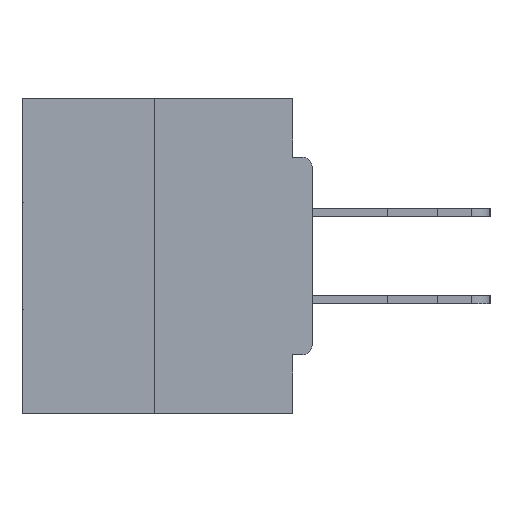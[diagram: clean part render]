
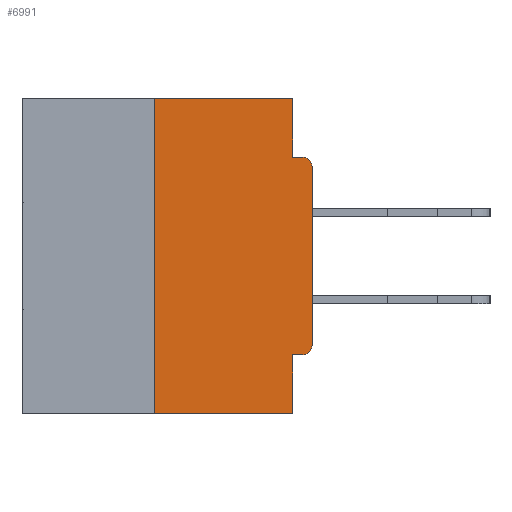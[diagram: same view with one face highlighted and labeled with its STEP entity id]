
A CAD part, left-side view. The second image highlights one B-rep face of the part: STEP entity #6991.
In plain terms, the highlighted planar face has unit normal (-1, 0, 0).
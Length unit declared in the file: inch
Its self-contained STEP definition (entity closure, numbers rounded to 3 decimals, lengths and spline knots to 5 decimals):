
#380 = CIRCLE ( 'NONE', #31904, 0.015 ) ;
#1742 = DIRECTION ( 'NONE',  ( 0., -1., 0. ) ) ;
#1920 = CARTESIAN_POINT ( 'NONE',  ( 0., 0.25, 0. ) ) ;
#2111 = DIRECTION ( 'NONE',  ( 0., 0., -1. ) ) ;
#2274 = LINE ( 'NONE', #31987, #38668 ) ;
#2423 = EDGE_CURVE ( 'NONE', #7994, #30855, #2274, .T. ) ;
#3061 = CARTESIAN_POINT ( 'NONE',  ( 0., 0., -0.4065 ) ) ;
#3167 = ORIENTED_EDGE ( 'NONE', *, *, #2423, .F. ) ;
#3292 = VERTEX_POINT ( 'NONE', #24908 ) ;
#3444 = ORIENTED_EDGE ( 'NONE', *, *, #24494, .T. ) ;
#4400 = EDGE_CURVE ( 'NONE', #24408, #22154, #13901, .T. ) ;
#4597 = CARTESIAN_POINT ( 'NONE',  ( 0., 0.46, -0.5 ) ) ;
#5049 = LINE ( 'NONE', #6935, #36256 ) ;
#5196 = CARTESIAN_POINT ( 'NONE',  ( 0., 0.015, -0.1085 ) ) ;
#6489 = AXIS2_PLACEMENT_3D ( 'NONE', #35710, #23314, #20119 ) ;
#6546 = CARTESIAN_POINT ( 'NONE',  ( 0., 0.031, 0. ) ) ;
#6935 = CARTESIAN_POINT ( 'NONE',  ( 0., 0.031, -0.5 ) ) ;
#6991 = ADVANCED_FACE ( 'NONE', ( #25486 ), #13376, .F. ) ;
#7063 = LINE ( 'NONE', #1920, #12255 ) ;
#7415 = EDGE_CURVE ( 'NONE', #3292, #23061, #25901, .T. ) ;
#7994 = VERTEX_POINT ( 'NONE', #30016 ) ;
#8171 = CARTESIAN_POINT ( 'NONE',  ( 0., 0.031, 0. ) ) ;
#8241 = CARTESIAN_POINT ( 'NONE',  ( 0., 0., -0.1085 ) ) ;
#8662 = VERTEX_POINT ( 'NONE', #27931 ) ;
#9055 = EDGE_LOOP ( 'NONE', ( #31337, #34740, #13455, #33193, #10926, #36842, #31069, #3444, #3167, #16853 ) ) ;
#9087 = EDGE_CURVE ( 'NONE', #8662, #24222, #30513, .T. ) ;
#9324 = EDGE_CURVE ( 'NONE', #22154, #23061, #5049, .T. ) ;
#10466 = DIRECTION ( 'NONE',  ( 0., 0., -1. ) ) ;
#10768 = CIRCLE ( 'NONE', #6489, 0.015 ) ;
#10926 = ORIENTED_EDGE ( 'NONE', *, *, #4400, .F. ) ;
#11288 = DIRECTION ( 'NONE',  ( -1., 0., 0. ) ) ;
#12234 = CARTESIAN_POINT ( 'NONE',  ( 0., 0.46, 0. ) ) ;
#12255 = VECTOR ( 'NONE', #34930, 39.37008 ) ;
#13376 = PLANE ( 'NONE',  #23803 ) ;
#13455 = ORIENTED_EDGE ( 'NONE', *, *, #7415, .T. ) ;
#13722 = VERTEX_POINT ( 'NONE', #32811 ) ;
#13901 = LINE ( 'NONE', #3061, #38012 ) ;
#14925 = DIRECTION ( 'NONE',  ( 0., 0., 1. ) ) ;
#15046 = CARTESIAN_POINT ( 'NONE',  ( 0., 0., 0. ) ) ;
#16214 = VECTOR ( 'NONE', #14925, 39.37008 ) ;
#16529 = CARTESIAN_POINT ( 'NONE',  ( 0., 0.46, 0. ) ) ;
#16853 = ORIENTED_EDGE ( 'NONE', *, *, #37909, .F. ) ;
#17855 = CARTESIAN_POINT ( 'NONE',  ( 0., 0.015, -0.0935 ) ) ;
#20119 = DIRECTION ( 'NONE',  ( 0., 0., -1. ) ) ;
#20407 = DIRECTION ( 'NONE',  ( 0., 0., -1. ) ) ;
#21419 = EDGE_CURVE ( 'NONE', #24408, #13722, #10768, .T. ) ;
#21556 = VECTOR ( 'NONE', #35613, 39.37008 ) ;
#22020 = CARTESIAN_POINT ( 'NONE',  ( 0., 0.015, -0.4065 ) ) ;
#22154 = VERTEX_POINT ( 'NONE', #23844 ) ;
#23061 = VERTEX_POINT ( 'NONE', #35053 ) ;
#23314 = DIRECTION ( 'NONE',  ( -1., 0., 0. ) ) ;
#23803 = AXIS2_PLACEMENT_3D ( 'NONE', #16529, #25124, #10466 ) ;
#23844 = CARTESIAN_POINT ( 'NONE',  ( 0., 0.031, -0.4065 ) ) ;
#24222 = VERTEX_POINT ( 'NONE', #6546 ) ;
#24339 = EDGE_CURVE ( 'NONE', #3292, #8662, #7063, .T. ) ;
#24408 = VERTEX_POINT ( 'NONE', #22020 ) ;
#24494 = EDGE_CURVE ( 'NONE', #27863, #30855, #380, .T. ) ;
#24908 = CARTESIAN_POINT ( 'NONE',  ( 0., 0.25, -0.5 ) ) ;
#25124 = DIRECTION ( 'NONE',  ( 1., 0., 0. ) ) ;
#25139 = DIRECTION ( 'NONE',  ( 0., 0., -1. ) ) ;
#25388 = LINE ( 'NONE', #8171, #37705 ) ;
#25486 = FACE_OUTER_BOUND ( 'NONE', #9055, .T. ) ;
#25841 = DIRECTION ( 'NONE',  ( 0., -1., 0. ) ) ;
#25901 = LINE ( 'NONE', #4597, #26394 ) ;
#26394 = VECTOR ( 'NONE', #25841, 39.37008 ) ;
#27863 = VERTEX_POINT ( 'NONE', #8241 ) ;
#27931 = CARTESIAN_POINT ( 'NONE',  ( 0., 0.25, 0. ) ) ;
#30016 = CARTESIAN_POINT ( 'NONE',  ( 0., 0.031, -0.0935 ) ) ;
#30388 = DIRECTION ( 'NONE',  ( 0., 1., 0. ) ) ;
#30513 = LINE ( 'NONE', #12234, #21556 ) ;
#30855 = VERTEX_POINT ( 'NONE', #17855 ) ;
#31069 = ORIENTED_EDGE ( 'NONE', *, *, #34678, .T. ) ;
#31337 = ORIENTED_EDGE ( 'NONE', *, *, #9087, .F. ) ;
#31904 = AXIS2_PLACEMENT_3D ( 'NONE', #5196, #11288, #20407 ) ;
#31987 = CARTESIAN_POINT ( 'NONE',  ( 0., 0., -0.0935 ) ) ;
#32281 = LINE ( 'NONE', #15046, #16214 ) ;
#32811 = CARTESIAN_POINT ( 'NONE',  ( 0., 0., -0.3915 ) ) ;
#33193 = ORIENTED_EDGE ( 'NONE', *, *, #9324, .F. ) ;
#34678 = EDGE_CURVE ( 'NONE', #13722, #27863, #32281, .T. ) ;
#34740 = ORIENTED_EDGE ( 'NONE', *, *, #24339, .F. ) ;
#34930 = DIRECTION ( 'NONE',  ( 0., 0., 1. ) ) ;
#35053 = CARTESIAN_POINT ( 'NONE',  ( 0., 0.031, -0.5 ) ) ;
#35613 = DIRECTION ( 'NONE',  ( 0., -1., 0. ) ) ;
#35710 = CARTESIAN_POINT ( 'NONE',  ( 0., 0.015, -0.3915 ) ) ;
#36256 = VECTOR ( 'NONE', #25139, 39.37008 ) ;
#36842 = ORIENTED_EDGE ( 'NONE', *, *, #21419, .T. ) ;
#37705 = VECTOR ( 'NONE', #2111, 39.37008 ) ;
#37909 = EDGE_CURVE ( 'NONE', #24222, #7994, #25388, .T. ) ;
#38012 = VECTOR ( 'NONE', #30388, 39.37008 ) ;
#38668 = VECTOR ( 'NONE', #1742, 39.37008 ) ;
